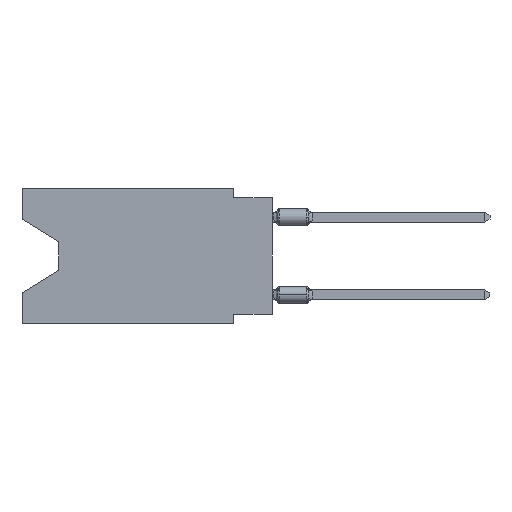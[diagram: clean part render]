
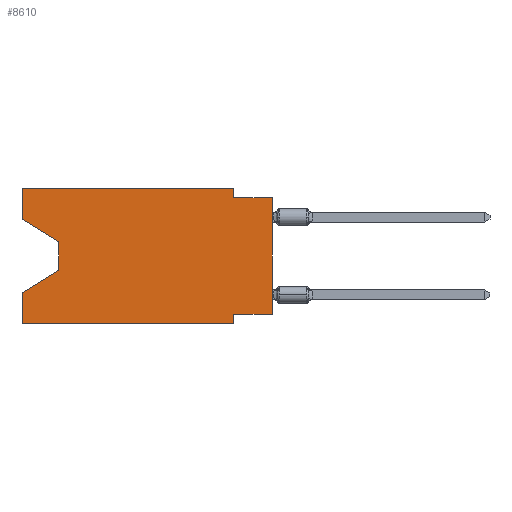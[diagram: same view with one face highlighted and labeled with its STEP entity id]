
A CAD part, left-side view. The second image highlights one B-rep face of the part: STEP entity #8610.
In plain terms, the highlighted planar face has unit normal (-1, 0, 0).
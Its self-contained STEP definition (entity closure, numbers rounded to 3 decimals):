
#555 = EDGE_CURVE ( 'NONE', #5586, #5606, #22882, .T. ) ;
#1001 = LINE ( 'NONE', #15160, #15324 ) ;
#1035 = LINE ( 'NONE', #18933, #1221 ) ;
#1221 = VECTOR ( 'NONE', #17163, 1000. ) ;
#1634 = CARTESIAN_POINT ( 'NONE',  ( 0., 13.97, -3.505 ) ) ;
#1927 = EDGE_CURVE ( 'NONE', #13928, #5586, #19273, .T. ) ;
#2454 = ORIENTED_EDGE ( 'NONE', *, *, #4998, .F. ) ;
#2527 = ORIENTED_EDGE ( 'NONE', *, *, #21384, .F. ) ;
#2575 = CARTESIAN_POINT ( 'NONE',  ( 0., 2.54, -0.635 ) ) ;
#2815 = VERTEX_POINT ( 'NONE', #18589 ) ;
#2822 = VERTEX_POINT ( 'NONE', #13116 ) ;
#2843 = DIRECTION ( 'NONE',  ( 0., 0.855, -0.519 ) ) ;
#2900 = DIRECTION ( 'NONE',  ( 0., -0.855, -0.519 ) ) ;
#3022 = LINE ( 'NONE', #17283, #16122 ) ;
#3090 = ORIENTED_EDGE ( 'NONE', *, *, #12860, .T. ) ;
#3113 = VECTOR ( 'NONE', #16240, 1000. ) ;
#3151 = VERTEX_POINT ( 'NONE', #19240 ) ;
#3348 = ORIENTED_EDGE ( 'NONE', *, *, #11743, .F. ) ;
#3782 = VECTOR ( 'NONE', #18295, 1000. ) ;
#4143 = VERTEX_POINT ( 'NONE', #22820 ) ;
#4233 = LINE ( 'NONE', #1634, #18965 ) ;
#4387 = ORIENTED_EDGE ( 'NONE', *, *, #5805, .T. ) ;
#4902 = AXIS2_PLACEMENT_3D ( 'NONE', #13830, #15361, #20982 ) ;
#4998 = EDGE_CURVE ( 'NONE', #2822, #22646, #17346, .T. ) ;
#5022 = ORIENTED_EDGE ( 'NONE', *, *, #12332, .T. ) ;
#5249 = CARTESIAN_POINT ( 'NONE',  ( 0., 0., 0. ) ) ;
#5335 = LINE ( 'NONE', #16078, #3782 ) ;
#5586 = VERTEX_POINT ( 'NONE', #11244 ) ;
#5606 = VERTEX_POINT ( 'NONE', #2575 ) ;
#5638 = EDGE_CURVE ( 'NONE', #2815, #13928, #1035, .T. ) ;
#5805 = EDGE_CURVE ( 'NONE', #2822, #7168, #10999, .T. ) ;
#6208 = CARTESIAN_POINT ( 'NONE',  ( 0., 0., -0.635 ) ) ;
#6574 = ORIENTED_EDGE ( 'NONE', *, *, #19657, .T. ) ;
#7168 = VERTEX_POINT ( 'NONE', #6208 ) ;
#7228 = CARTESIAN_POINT ( 'NONE',  ( 0., 2.54, -8.255 ) ) ;
#7332 = LINE ( 'NONE', #12496, #18971 ) ;
#7939 = VECTOR ( 'NONE', #8451, 1000. ) ;
#8451 = DIRECTION ( 'NONE',  ( 0., 1., 0. ) ) ;
#8610 = ADVANCED_FACE ( 'NONE', ( #12198 ), #15575, .F. ) ;
#10317 = EDGE_LOOP ( 'NONE', ( #5022, #6574, #12573, #15778, #3090, #3348, #2454, #4387, #2527, #15451, #12434, #11516 ) ) ;
#10999 = LINE ( 'NONE', #5249, #3113 ) ;
#11182 = DIRECTION ( 'NONE',  ( 0., -1., 0. ) ) ;
#11244 = CARTESIAN_POINT ( 'NONE',  ( 0., 2.54, 0. ) ) ;
#11516 = ORIENTED_EDGE ( 'NONE', *, *, #5638, .F. ) ;
#11743 = EDGE_CURVE ( 'NONE', #22646, #18275, #5335, .T. ) ;
#11904 = LINE ( 'NONE', #15863, #19755 ) ;
#12162 = CARTESIAN_POINT ( 'NONE',  ( 0., 13.97, -3.505 ) ) ;
#12198 = FACE_OUTER_BOUND ( 'NONE', #10317, .T. ) ;
#12332 = EDGE_CURVE ( 'NONE', #2815, #22137, #3022, .T. ) ;
#12355 = DIRECTION ( 'NONE',  ( 0., 0., -1. ) ) ;
#12434 = ORIENTED_EDGE ( 'NONE', *, *, #1927, .F. ) ;
#12496 = CARTESIAN_POINT ( 'NONE',  ( 0., 0., -0.635 ) ) ;
#12573 = ORIENTED_EDGE ( 'NONE', *, *, #22956, .T. ) ;
#12860 = EDGE_CURVE ( 'NONE', #15593, #18275, #1001, .T. ) ;
#12950 = DIRECTION ( 'NONE',  ( 0., -1., 0. ) ) ;
#13116 = CARTESIAN_POINT ( 'NONE',  ( 0., 0., -8.255 ) ) ;
#13634 = DIRECTION ( 'NONE',  ( 0., -1., 0. ) ) ;
#13830 = CARTESIAN_POINT ( 'NONE',  ( 0., 16.383, 0. ) ) ;
#13928 = VERTEX_POINT ( 'NONE', #22644 ) ;
#14543 = CARTESIAN_POINT ( 'NONE',  ( 0., 2.54, -8.89 ) ) ;
#15126 = CARTESIAN_POINT ( 'NONE',  ( 0., 13.97, -5.385 ) ) ;
#15160 = CARTESIAN_POINT ( 'NONE',  ( 0., 16.383, -8.89 ) ) ;
#15324 = VECTOR ( 'NONE', #13634, 1000. ) ;
#15361 = DIRECTION ( 'NONE',  ( 1., 0., 0. ) ) ;
#15451 = ORIENTED_EDGE ( 'NONE', *, *, #555, .F. ) ;
#15457 = VECTOR ( 'NONE', #11182, 1000. ) ;
#15505 = CARTESIAN_POINT ( 'NONE',  ( 0., 2.54, 0. ) ) ;
#15575 = PLANE ( 'NONE',  #4902 ) ;
#15593 = VERTEX_POINT ( 'NONE', #15791 ) ;
#15777 = DIRECTION ( 'NONE',  ( 0., 0., -1. ) ) ;
#15778 = ORIENTED_EDGE ( 'NONE', *, *, #22560, .F. ) ;
#15786 = VECTOR ( 'NONE', #12355, 1000. ) ;
#15791 = CARTESIAN_POINT ( 'NONE',  ( 0., 16.383, -8.89 ) ) ;
#15826 = CARTESIAN_POINT ( 'NONE',  ( 0., 0., -8.255 ) ) ;
#15863 = CARTESIAN_POINT ( 'NONE',  ( 0., 16.383, 0. ) ) ;
#16078 = CARTESIAN_POINT ( 'NONE',  ( 0., 2.54, -8.89 ) ) ;
#16122 = VECTOR ( 'NONE', #2900, 1000. ) ;
#16240 = DIRECTION ( 'NONE',  ( 0., 0., 1. ) ) ;
#17163 = DIRECTION ( 'NONE',  ( 0., 0., 1. ) ) ;
#17283 = CARTESIAN_POINT ( 'NONE',  ( 0., 16.383, -2.038 ) ) ;
#17346 = LINE ( 'NONE', #15826, #7939 ) ;
#18088 = CARTESIAN_POINT ( 'NONE',  ( 0., 16.383, 0. ) ) ;
#18275 = VERTEX_POINT ( 'NONE', #14543 ) ;
#18295 = DIRECTION ( 'NONE',  ( 0., 0., -1. ) ) ;
#18589 = CARTESIAN_POINT ( 'NONE',  ( 0., 16.383, -2.038 ) ) ;
#18933 = CARTESIAN_POINT ( 'NONE',  ( 0., 16.383, 0. ) ) ;
#18965 = VECTOR ( 'NONE', #15777, 1000. ) ;
#18971 = VECTOR ( 'NONE', #12950, 1000. ) ;
#19240 = CARTESIAN_POINT ( 'NONE',  ( 0., 13.97, -5.385 ) ) ;
#19273 = LINE ( 'NONE', #18088, #15457 ) ;
#19315 = VECTOR ( 'NONE', #2843, 1000. ) ;
#19502 = DIRECTION ( 'NONE',  ( 0., 0., 1. ) ) ;
#19657 = EDGE_CURVE ( 'NONE', #22137, #3151, #4233, .T. ) ;
#19755 = VECTOR ( 'NONE', #19502, 1000. ) ;
#20509 = LINE ( 'NONE', #15126, #19315 ) ;
#20982 = DIRECTION ( 'NONE',  ( 0., 0., -1. ) ) ;
#21384 = EDGE_CURVE ( 'NONE', #5606, #7168, #7332, .T. ) ;
#22137 = VERTEX_POINT ( 'NONE', #12162 ) ;
#22560 = EDGE_CURVE ( 'NONE', #15593, #4143, #11904, .T. ) ;
#22644 = CARTESIAN_POINT ( 'NONE',  ( 0., 16.383, 0. ) ) ;
#22646 = VERTEX_POINT ( 'NONE', #7228 ) ;
#22820 = CARTESIAN_POINT ( 'NONE',  ( 0., 16.383, -6.852 ) ) ;
#22882 = LINE ( 'NONE', #15505, #15786 ) ;
#22956 = EDGE_CURVE ( 'NONE', #3151, #4143, #20509, .T. ) ;
